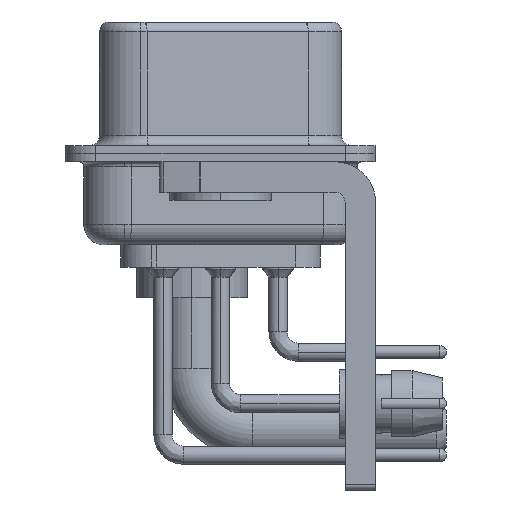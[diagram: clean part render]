
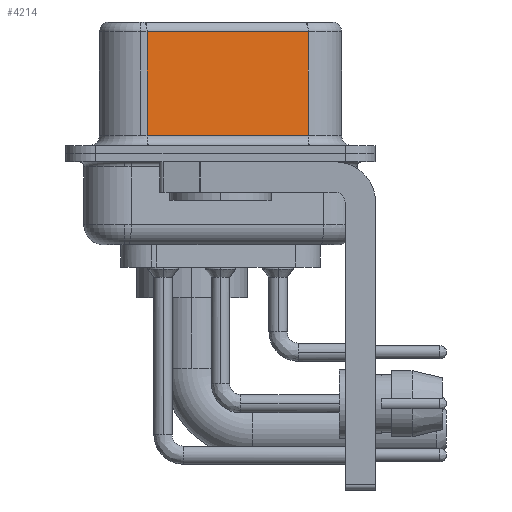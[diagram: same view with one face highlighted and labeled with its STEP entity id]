
A CAD part, left-side view. The second image highlights one B-rep face of the part: STEP entity #4214.
In plain terms, the highlighted planar face has unit normal (-0.985, -0.174, 0).
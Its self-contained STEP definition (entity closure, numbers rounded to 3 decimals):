
#409 = ORIENTED_EDGE ( 'NONE', *, *, #37450, .T. ) ;
#2017 = ORIENTED_EDGE ( 'NONE', *, *, #14893, .F. ) ;
#2711 = EDGE_CURVE ( 'NONE', #5623, #26051, #30808, .T. ) ;
#3169 = LINE ( 'NONE', #24091, #4036 ) ;
#3340 = PLANE ( 'NONE',  #10515 ) ;
#4036 = VECTOR ( 'NONE', #36017, 1000. ) ;
#4214 = ADVANCED_FACE ( 'NONE', ( #29568 ), #3340, .F. ) ;
#4511 = CARTESIAN_POINT ( 'NONE',  ( 3.73, 3.628, 0.9 ) ) ;
#5395 = DIRECTION ( 'NONE',  ( -0.174, 0.985, 0. ) ) ;
#5623 = VERTEX_POINT ( 'NONE', #4511 ) ;
#9226 = DIRECTION ( 'NONE',  ( 0.985, 0.174, 0. ) ) ;
#9363 = LINE ( 'NONE', #18542, #17966 ) ;
#10515 = AXIS2_PLACEMENT_3D ( 'NONE', #14506, #9226, #11783 ) ;
#11783 = DIRECTION ( 'NONE',  ( -0.174, 0.985, 0. ) ) ;
#14506 = CARTESIAN_POINT ( 'NONE',  ( 5.132, -4.322, 6.52 ) ) ;
#14893 = EDGE_CURVE ( 'NONE', #33765, #26051, #9363, .T. ) ;
#16277 = ORIENTED_EDGE ( 'NONE', *, *, #2711, .T. ) ;
#17966 = VECTOR ( 'NONE', #30283, 1000. ) ;
#18542 = CARTESIAN_POINT ( 'NONE',  ( 5.132, -4.322, 6.52 ) ) ;
#19301 = ORIENTED_EDGE ( 'NONE', *, *, #28585, .T. ) ;
#20236 = LINE ( 'NONE', #35105, #33756 ) ;
#21465 = CARTESIAN_POINT ( 'NONE',  ( 3.73, 3.628, 6.02 ) ) ;
#24091 = CARTESIAN_POINT ( 'NONE',  ( 3.73, 3.628, 6.52 ) ) ;
#26051 = VERTEX_POINT ( 'NONE', #33066 ) ;
#26568 = VERTEX_POINT ( 'NONE', #21465 ) ;
#28585 = EDGE_CURVE ( 'NONE', #26568, #5623, #3169, .T. ) ;
#29568 = FACE_OUTER_BOUND ( 'NONE', #31493, .T. ) ;
#29708 = DIRECTION ( 'NONE',  ( 0.174, -0.985, 0. ) ) ;
#30283 = DIRECTION ( 'NONE',  ( 0., 0., -1. ) ) ;
#30808 = LINE ( 'NONE', #35583, #33503 ) ;
#31460 = CARTESIAN_POINT ( 'NONE',  ( 5.132, -4.322, 6.02 ) ) ;
#31493 = EDGE_LOOP ( 'NONE', ( #2017, #409, #19301, #16277 ) ) ;
#33066 = CARTESIAN_POINT ( 'NONE',  ( 5.132, -4.322, 0.9 ) ) ;
#33503 = VECTOR ( 'NONE', #29708, 1000. ) ;
#33756 = VECTOR ( 'NONE', #5395, 1000. ) ;
#33765 = VERTEX_POINT ( 'NONE', #31460 ) ;
#35105 = CARTESIAN_POINT ( 'NONE',  ( 5.132, -4.322, 6.02 ) ) ;
#35583 = CARTESIAN_POINT ( 'NONE',  ( 5.132, -4.322, 0.9 ) ) ;
#36017 = DIRECTION ( 'NONE',  ( 0., 0., -1. ) ) ;
#37450 = EDGE_CURVE ( 'NONE', #33765, #26568, #20236, .T. ) ;
